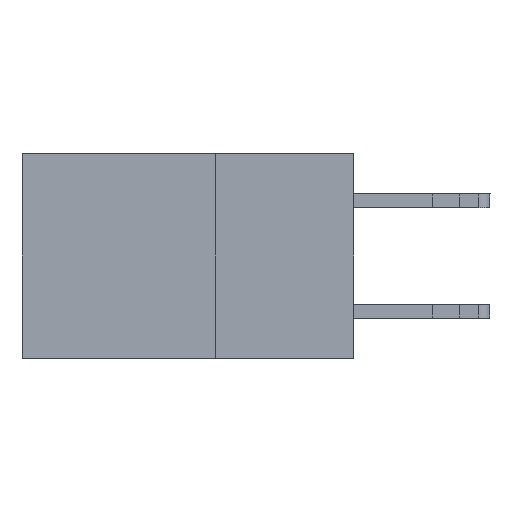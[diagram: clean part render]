
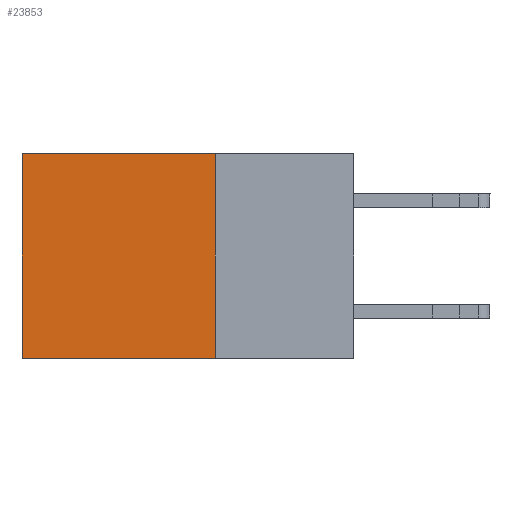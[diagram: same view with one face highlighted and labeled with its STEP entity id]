
A CAD part, left-side view. The second image highlights one B-rep face of the part: STEP entity #23853.
In plain terms, the highlighted planar face has unit normal (-1, 0, 0).
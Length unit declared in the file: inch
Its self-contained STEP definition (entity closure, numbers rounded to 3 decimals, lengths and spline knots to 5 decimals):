
#457 = CARTESIAN_POINT ( 'NONE',  ( 0.2875, 0.6, 0. ) ) ;
#577 = CARTESIAN_POINT ( 'NONE',  ( 0.2875, 0.25, 0. ) ) ;
#2304 = CARTESIAN_POINT ( 'NONE',  ( 0.2875, 0.25, 0. ) ) ;
#2826 = DIRECTION ( 'NONE',  ( 1., 0., 0. ) ) ;
#4609 = EDGE_CURVE ( 'NONE', #31449, #9595, #32413, .T. ) ;
#5141 = EDGE_CURVE ( 'NONE', #31449, #13504, #24594, .T. ) ;
#5587 = VECTOR ( 'NONE', #31617, 39.37008 ) ;
#6456 = CARTESIAN_POINT ( 'NONE',  ( 0.2875, 0.6, 0. ) ) ;
#8052 = CARTESIAN_POINT ( 'NONE',  ( 0.2875, 0.25, -0.37 ) ) ;
#8344 = DIRECTION ( 'NONE',  ( 0., 1., 0. ) ) ;
#8433 = DIRECTION ( 'NONE',  ( 0., 0., -1. ) ) ;
#8800 = AXIS2_PLACEMENT_3D ( 'NONE', #11107, #2826, #8433 ) ;
#9595 = VERTEX_POINT ( 'NONE', #457 ) ;
#11107 = CARTESIAN_POINT ( 'NONE',  ( 0.2875, 0.25, 0. ) ) ;
#11504 = CARTESIAN_POINT ( 'NONE',  ( 0.2875, 0.25, -0.37 ) ) ;
#13198 = LINE ( 'NONE', #11504, #22785 ) ;
#13504 = VERTEX_POINT ( 'NONE', #8052 ) ;
#19059 = ORIENTED_EDGE ( 'NONE', *, *, #5141, .F. ) ;
#19979 = ORIENTED_EDGE ( 'NONE', *, *, #32905, .T. ) ;
#20828 = LINE ( 'NONE', #6456, #5587 ) ;
#21998 = PLANE ( 'NONE',  #8800 ) ;
#22785 = VECTOR ( 'NONE', #8344, 39.37008 ) ;
#23139 = EDGE_CURVE ( 'NONE', #13504, #30573, #13198, .T. ) ;
#23853 = ADVANCED_FACE ( 'NONE', ( #31478 ), #21998, .F. ) ;
#24594 = LINE ( 'NONE', #577, #28518 ) ;
#25259 = ORIENTED_EDGE ( 'NONE', *, *, #23139, .F. ) ;
#25755 = DIRECTION ( 'NONE',  ( 0., 0., -1. ) ) ;
#26721 = VECTOR ( 'NONE', #35313, 39.37008 ) ;
#28518 = VECTOR ( 'NONE', #25755, 39.37008 ) ;
#29950 = CARTESIAN_POINT ( 'NONE',  ( 0.2875, 0.25, 0. ) ) ;
#30573 = VERTEX_POINT ( 'NONE', #34092 ) ;
#31449 = VERTEX_POINT ( 'NONE', #2304 ) ;
#31478 = FACE_OUTER_BOUND ( 'NONE', #33697, .T. ) ;
#31617 = DIRECTION ( 'NONE',  ( 0., 0., -1. ) ) ;
#31863 = ORIENTED_EDGE ( 'NONE', *, *, #4609, .T. ) ;
#32413 = LINE ( 'NONE', #29950, #26721 ) ;
#32905 = EDGE_CURVE ( 'NONE', #9595, #30573, #20828, .T. ) ;
#33697 = EDGE_LOOP ( 'NONE', ( #19979, #25259, #19059, #31863 ) ) ;
#34092 = CARTESIAN_POINT ( 'NONE',  ( 0.2875, 0.6, -0.37 ) ) ;
#35313 = DIRECTION ( 'NONE',  ( 0., 1., 0. ) ) ;
